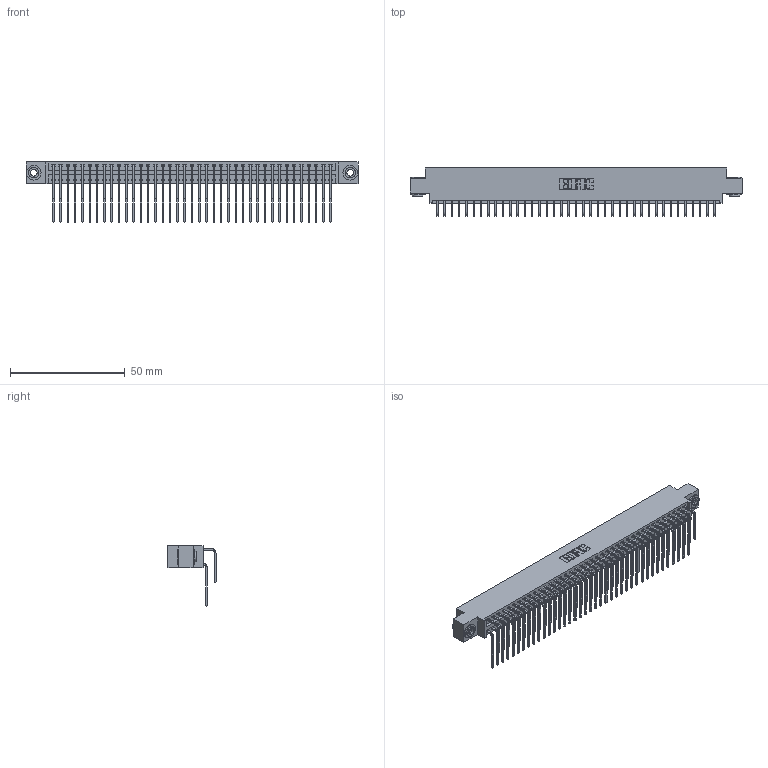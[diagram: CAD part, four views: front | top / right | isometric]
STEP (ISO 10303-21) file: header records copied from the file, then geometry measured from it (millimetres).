
FILE_DESCRIPTION (( 'STEP AP203' ), '1' );
FILE_NAME ('346-078-559-803.STEP', '2022-05-25T14:50:57', ( '' ), ( '' ), 'SwSTEP 2.0', 'SolidWorks 2020', '' );
FILE_SCHEMA (( 'CONFIG_CONTROL_DESIGN' ));
Length unit declared in the file: inch
Products named in the file (5): 346-078-559-803; 346 Part_0.170 Offset - 0.156 Dia-TH; 345-250-002_345-250-002-102; 345-292-001_558 559 Tail - 1; 345-292-001_559 Tail - 2
Assembly tree (81 placements, depth 2):
  346-078-559-803
    346 Part_0.170 Offset - 0.156 Dia-TH
    345-292-001_558 559 Tail - 1  x39
    345-292-001_559 Tail - 2  x39
    345-250-002_345-250-002-102  x2
Bounding box: 144.4 x 20.89 x 26.16 mm (x, y, z)
Volume: 14354 mm3; surface area: 22270.4 mm2
Topology: 81 solids, 81 shells, 4390 faces, 13011 edges, 8566 vertices
Faces by surface type: plane 2990, cylinder 1392, cone 8
Entity records: 28838 total; most frequent: CARTESIAN_POINT 4792, ORIENTED_EDGE 4666, DIRECTION 4275, EDGE_CURVE 2333, LINE 1981, VECTOR 1981, VERTEX_POINT 1550, AXIS2_PLACEMENT_3D 1147
